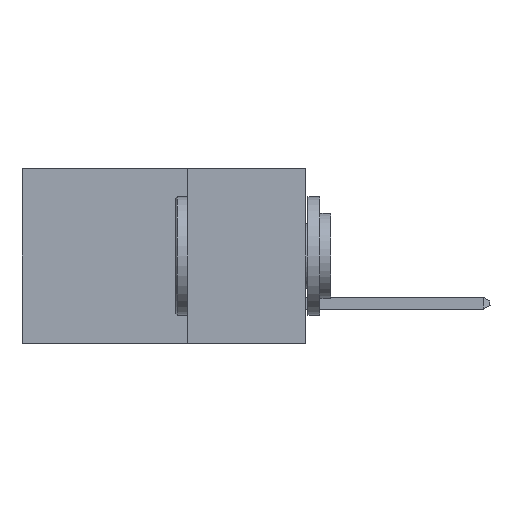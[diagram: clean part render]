
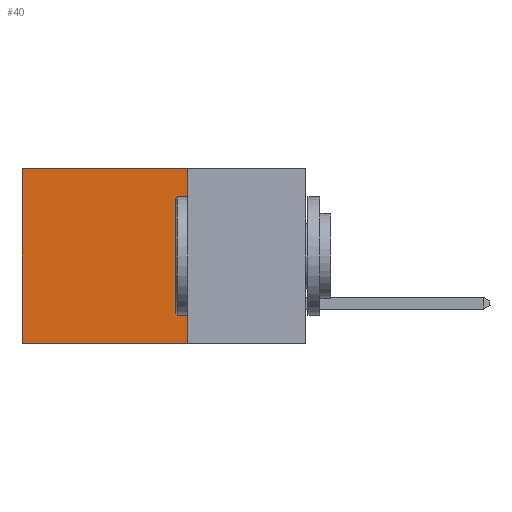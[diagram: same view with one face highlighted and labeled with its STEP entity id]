
A CAD part, left-side view. The second image highlights one B-rep face of the part: STEP entity #40.
In plain terms, the highlighted planar face has unit normal (-1, 0, 0).
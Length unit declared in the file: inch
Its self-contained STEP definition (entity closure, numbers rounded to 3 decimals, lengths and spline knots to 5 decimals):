
#40 = ADVANCED_FACE ( 'NONE', ( #7398 ), #3135, .F. ) ;
#325 = EDGE_CURVE ( 'NONE', #6503, #1453, #3275, .T. ) ;
#398 = EDGE_CURVE ( 'NONE', #1453, #3729, #4586, .T. ) ;
#445 = DIRECTION ( 'NONE',  ( 0., 1., 0. ) ) ;
#1453 = VERTEX_POINT ( 'NONE', #9821 ) ;
#2030 = EDGE_CURVE ( 'NONE', #10282, #3729, #8313, .T. ) ;
#2308 = VECTOR ( 'NONE', #7190, 39.37008 ) ;
#2685 = VECTOR ( 'NONE', #8404, 39.37008 ) ;
#2837 = CARTESIAN_POINT ( 'NONE',  ( 0.298, 0.25, 0. ) ) ;
#3135 = PLANE ( 'NONE',  #4820 ) ;
#3275 = LINE ( 'NONE', #7732, #7390 ) ;
#3329 = EDGE_CURVE ( 'NONE', #6503, #10282, #5109, .T. ) ;
#3729 = VERTEX_POINT ( 'NONE', #3807 ) ;
#3807 = CARTESIAN_POINT ( 'NONE',  ( 0.298, 0.6, -0.37 ) ) ;
#4586 = LINE ( 'NONE', #8452, #2685 ) ;
#4792 = CARTESIAN_POINT ( 'NONE',  ( 0.298, 0.25, 0. ) ) ;
#4820 = AXIS2_PLACEMENT_3D ( 'NONE', #4792, #5784, #6852 ) ;
#5109 = LINE ( 'NONE', #5303, #2308 ) ;
#5303 = CARTESIAN_POINT ( 'NONE',  ( 0.298, 0.25, 0. ) ) ;
#5784 = DIRECTION ( 'NONE',  ( 1., 0., 0. ) ) ;
#6180 = VECTOR ( 'NONE', #445, 39.37008 ) ;
#6503 = VERTEX_POINT ( 'NONE', #2837 ) ;
#6852 = DIRECTION ( 'NONE',  ( 0., 0., -1. ) ) ;
#6984 = CARTESIAN_POINT ( 'NONE',  ( 0.298, 0.25, -0.37 ) ) ;
#7190 = DIRECTION ( 'NONE',  ( 0., 0., -1. ) ) ;
#7390 = VECTOR ( 'NONE', #10276, 39.37008 ) ;
#7398 = FACE_OUTER_BOUND ( 'NONE', #8592, .T. ) ;
#7643 = ORIENTED_EDGE ( 'NONE', *, *, #398, .T. ) ;
#7732 = CARTESIAN_POINT ( 'NONE',  ( 0.298, 0.25, 0. ) ) ;
#8030 = CARTESIAN_POINT ( 'NONE',  ( 0.298, 0.25, -0.37 ) ) ;
#8313 = LINE ( 'NONE', #8030, #6180 ) ;
#8404 = DIRECTION ( 'NONE',  ( 0., 0., -1. ) ) ;
#8452 = CARTESIAN_POINT ( 'NONE',  ( 0.298, 0.6, 0. ) ) ;
#8592 = EDGE_LOOP ( 'NONE', ( #7643, #8796, #9629, #10066 ) ) ;
#8796 = ORIENTED_EDGE ( 'NONE', *, *, #2030, .F. ) ;
#9629 = ORIENTED_EDGE ( 'NONE', *, *, #3329, .F. ) ;
#9821 = CARTESIAN_POINT ( 'NONE',  ( 0.298, 0.6, 0. ) ) ;
#10066 = ORIENTED_EDGE ( 'NONE', *, *, #325, .T. ) ;
#10276 = DIRECTION ( 'NONE',  ( 0., 1., 0. ) ) ;
#10282 = VERTEX_POINT ( 'NONE', #6984 ) ;
